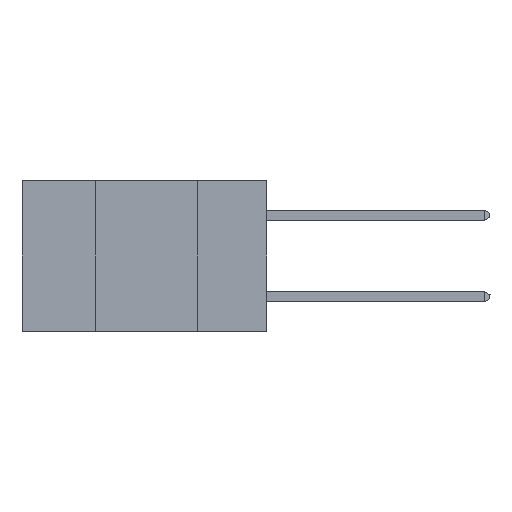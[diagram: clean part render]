
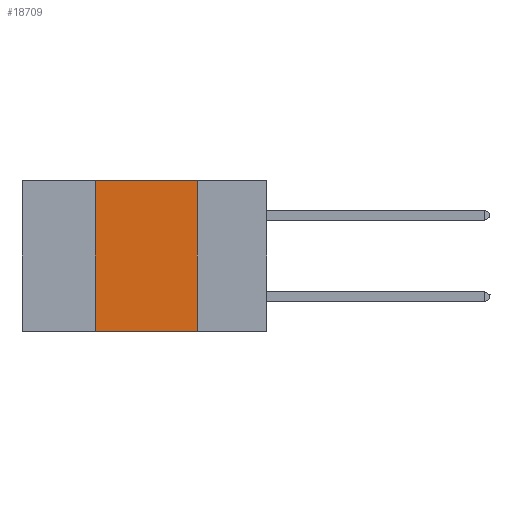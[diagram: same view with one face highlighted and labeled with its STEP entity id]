
A CAD part, left-side view. The second image highlights one B-rep face of the part: STEP entity #18709.
In plain terms, the highlighted planar face has unit normal (-1, 0, 0).
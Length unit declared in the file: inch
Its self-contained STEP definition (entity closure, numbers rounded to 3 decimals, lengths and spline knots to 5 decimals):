
#298 = CARTESIAN_POINT ( 'NONE',  ( 0., 0.42, 0. ) ) ;
#365 = VECTOR ( 'NONE', #15601, 39.37008 ) ;
#2676 = LINE ( 'NONE', #3043, #365 ) ;
#3043 = CARTESIAN_POINT ( 'NONE',  ( 0., 0.6, 0. ) ) ;
#3367 = CARTESIAN_POINT ( 'NONE',  ( 0., 0.17, 0. ) ) ;
#3911 = ORIENTED_EDGE ( 'NONE', *, *, #14455, .T. ) ;
#4293 = PLANE ( 'NONE',  #13727 ) ;
#4492 = CARTESIAN_POINT ( 'NONE',  ( 0., 0.42, -0.37 ) ) ;
#4964 = ORIENTED_EDGE ( 'NONE', *, *, #11252, .F. ) ;
#5420 = CARTESIAN_POINT ( 'NONE',  ( 0., 0.6, -0.37 ) ) ;
#6056 = ORIENTED_EDGE ( 'NONE', *, *, #10788, .F. ) ;
#6077 = LINE ( 'NONE', #5420, #9730 ) ;
#6642 = VERTEX_POINT ( 'NONE', #7730 ) ;
#7067 = VERTEX_POINT ( 'NONE', #15406 ) ;
#7530 = DIRECTION ( 'NONE',  ( 0., 0., 1. ) ) ;
#7730 = CARTESIAN_POINT ( 'NONE',  ( 0., 0.42, 0. ) ) ;
#7926 = DIRECTION ( 'NONE',  ( 1., 0., 0. ) ) ;
#9730 = VECTOR ( 'NONE', #19988, 39.37008 ) ;
#9732 = DIRECTION ( 'NONE',  ( 0., 0., -1. ) ) ;
#9865 = FACE_OUTER_BOUND ( 'NONE', #10533, .T. ) ;
#10533 = EDGE_LOOP ( 'NONE', ( #4964, #22380, #6056, #3911 ) ) ;
#10788 = EDGE_CURVE ( 'NONE', #15935, #6642, #21772, .T. ) ;
#11252 = EDGE_CURVE ( 'NONE', #15936, #7067, #12400, .T. ) ;
#12173 = DIRECTION ( 'NONE',  ( 0., 0., -1. ) ) ;
#12400 = LINE ( 'NONE', #3367, #18622 ) ;
#13727 = AXIS2_PLACEMENT_3D ( 'NONE', #18510, #7926, #9732 ) ;
#14455 = EDGE_CURVE ( 'NONE', #15935, #7067, #6077, .T. ) ;
#15393 = EDGE_CURVE ( 'NONE', #6642, #15936, #2676, .T. ) ;
#15406 = CARTESIAN_POINT ( 'NONE',  ( 0., 0.17, -0.37 ) ) ;
#15601 = DIRECTION ( 'NONE',  ( 0., -1., 0. ) ) ;
#15935 = VERTEX_POINT ( 'NONE', #4492 ) ;
#15936 = VERTEX_POINT ( 'NONE', #19175 ) ;
#16965 = VECTOR ( 'NONE', #7530, 39.37008 ) ;
#18510 = CARTESIAN_POINT ( 'NONE',  ( 0., 0.6, 0. ) ) ;
#18622 = VECTOR ( 'NONE', #12173, 39.37008 ) ;
#18709 = ADVANCED_FACE ( 'NONE', ( #9865 ), #4293, .F. ) ;
#19175 = CARTESIAN_POINT ( 'NONE',  ( 0., 0.17, 0. ) ) ;
#19988 = DIRECTION ( 'NONE',  ( 0., -1., 0. ) ) ;
#21772 = LINE ( 'NONE', #298, #16965 ) ;
#22380 = ORIENTED_EDGE ( 'NONE', *, *, #15393, .F. ) ;
